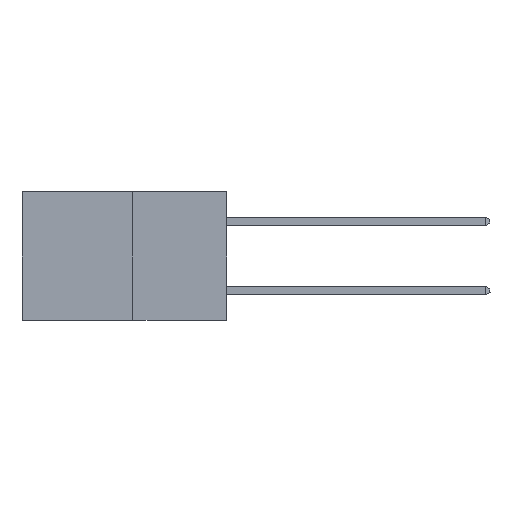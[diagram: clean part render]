
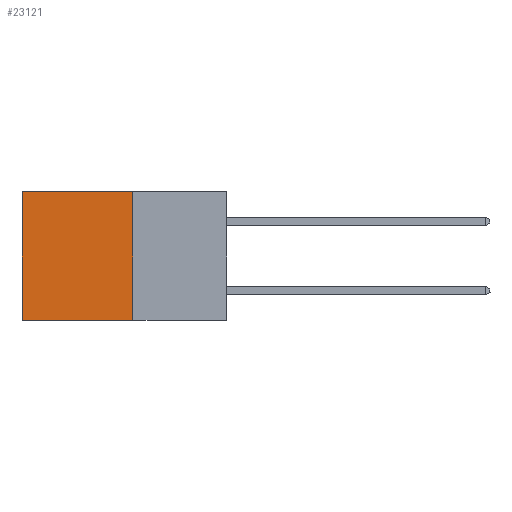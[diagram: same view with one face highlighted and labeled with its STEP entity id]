
A CAD part, left-side view. The second image highlights one B-rep face of the part: STEP entity #23121.
In plain terms, the highlighted planar face has unit normal (-1, 0, 0).
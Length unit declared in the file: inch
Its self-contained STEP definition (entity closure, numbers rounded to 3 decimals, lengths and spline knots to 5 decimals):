
#1226 = EDGE_LOOP ( 'NONE', ( #14878, #19309, #6260, #2337 ) ) ;
#1669 = VERTEX_POINT ( 'NONE', #14419 ) ;
#1693 = CARTESIAN_POINT ( 'NONE',  ( 0.277, 0.59, -0.37 ) ) ;
#1966 = LINE ( 'NONE', #17928, #22208 ) ;
#2337 = ORIENTED_EDGE ( 'NONE', *, *, #24613, .T. ) ;
#2890 = CARTESIAN_POINT ( 'NONE',  ( 0.277, 0.27, -0.37 ) ) ;
#4103 = CARTESIAN_POINT ( 'NONE',  ( 0.277, 0.27, -0.37 ) ) ;
#4504 = LINE ( 'NONE', #23064, #19442 ) ;
#4860 = VECTOR ( 'NONE', #15428, 39.37008 ) ;
#4905 = DIRECTION ( 'NONE',  ( 0., 0., -1. ) ) ;
#5993 = FACE_OUTER_BOUND ( 'NONE', #1226, .T. ) ;
#6260 = ORIENTED_EDGE ( 'NONE', *, *, #11479, .F. ) ;
#7102 = AXIS2_PLACEMENT_3D ( 'NONE', #2890, #16597, #4905 ) ;
#8288 = DIRECTION ( 'NONE',  ( 0., 1., 0. ) ) ;
#10135 = LINE ( 'NONE', #13489, #4860 ) ;
#10517 = CARTESIAN_POINT ( 'NONE',  ( 0.277, 0.27, 0. ) ) ;
#11479 = EDGE_CURVE ( 'NONE', #14707, #20883, #10135, .T. ) ;
#11764 = VECTOR ( 'NONE', #15469, 39.37008 ) ;
#12393 = LINE ( 'NONE', #1693, #11764 ) ;
#13489 = CARTESIAN_POINT ( 'NONE',  ( 0.277, 0.27, -0.37 ) ) ;
#14419 = CARTESIAN_POINT ( 'NONE',  ( 0.277, 0.59, -0.37 ) ) ;
#14707 = VERTEX_POINT ( 'NONE', #10517 ) ;
#14878 = ORIENTED_EDGE ( 'NONE', *, *, #15142, .T. ) ;
#15142 = EDGE_CURVE ( 'NONE', #19511, #1669, #12393, .T. ) ;
#15428 = DIRECTION ( 'NONE',  ( 0., 0., -1. ) ) ;
#15469 = DIRECTION ( 'NONE',  ( 0., 0., -1. ) ) ;
#16494 = CARTESIAN_POINT ( 'NONE',  ( 0.277, 0.59, 0. ) ) ;
#16597 = DIRECTION ( 'NONE',  ( 1., 0., 0. ) ) ;
#17290 = DIRECTION ( 'NONE',  ( 0., 1., 0. ) ) ;
#17928 = CARTESIAN_POINT ( 'NONE',  ( 0.277, 0.27, -0.37 ) ) ;
#19309 = ORIENTED_EDGE ( 'NONE', *, *, #21665, .F. ) ;
#19442 = VECTOR ( 'NONE', #17290, 39.37008 ) ;
#19511 = VERTEX_POINT ( 'NONE', #16494 ) ;
#20883 = VERTEX_POINT ( 'NONE', #4103 ) ;
#21665 = EDGE_CURVE ( 'NONE', #20883, #1669, #1966, .T. ) ;
#22208 = VECTOR ( 'NONE', #8288, 39.37008 ) ;
#23064 = CARTESIAN_POINT ( 'NONE',  ( 0.277, 0.27, 0. ) ) ;
#23121 = ADVANCED_FACE ( 'NONE', ( #5993 ), #24318, .F. ) ;
#24318 = PLANE ( 'NONE',  #7102 ) ;
#24613 = EDGE_CURVE ( 'NONE', #14707, #19511, #4504, .T. ) ;
